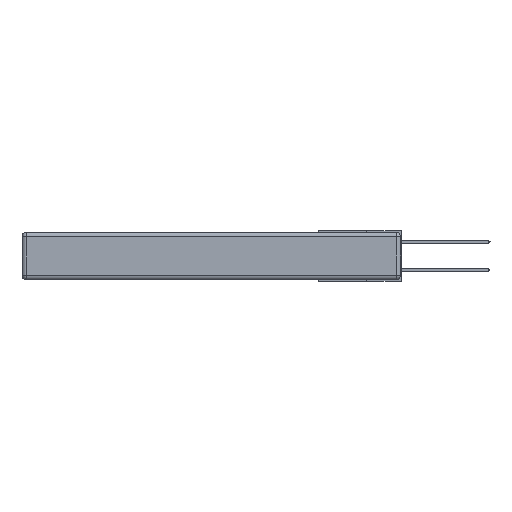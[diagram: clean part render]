
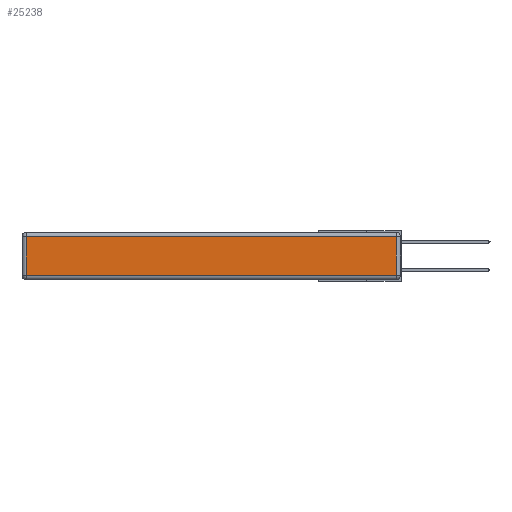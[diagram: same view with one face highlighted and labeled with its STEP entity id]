
A CAD part, left-side view. The second image highlights one B-rep face of the part: STEP entity #25238.
In plain terms, the highlighted planar face has unit normal (-1, 0, 0).
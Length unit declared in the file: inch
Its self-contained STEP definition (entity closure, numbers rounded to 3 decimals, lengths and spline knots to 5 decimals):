
#704 = AXIS2_PLACEMENT_3D ( 'NONE', #15070, #11145, #9154 ) ;
#1471 = VERTEX_POINT ( 'NONE', #9266 ) ;
#2632 = EDGE_LOOP ( 'NONE', ( #19724, #6106, #23826, #5443 ) ) ;
#4002 = VECTOR ( 'NONE', #16890, 39.37008 ) ;
#4607 = LINE ( 'NONE', #25486, #22630 ) ;
#4851 = CARTESIAN_POINT ( 'NONE',  ( 0., 2.72, -0.343 ) ) ;
#5285 = CARTESIAN_POINT ( 'NONE',  ( 0., 2.72, -0.03 ) ) ;
#5443 = ORIENTED_EDGE ( 'NONE', *, *, #9253, .T. ) ;
#6106 = ORIENTED_EDGE ( 'NONE', *, *, #17578, .T. ) ;
#6885 = DIRECTION ( 'NONE',  ( 0., 0., 1. ) ) ;
#8106 = DIRECTION ( 'NONE',  ( 0., 1., 0. ) ) ;
#9154 = DIRECTION ( 'NONE',  ( 0., 0., 1. ) ) ;
#9253 = EDGE_CURVE ( 'NONE', #11743, #22952, #15229, .T. ) ;
#9266 = CARTESIAN_POINT ( 'NONE',  ( 0., 0.03, -0.313 ) ) ;
#11145 = DIRECTION ( 'NONE',  ( -1., 0., 0. ) ) ;
#11191 = EDGE_CURVE ( 'NONE', #17053, #11743, #20093, .T. ) ;
#11743 = VERTEX_POINT ( 'NONE', #5285 ) ;
#13769 = CARTESIAN_POINT ( 'NONE',  ( 0., 0.03, -0.03 ) ) ;
#13907 = VECTOR ( 'NONE', #6885, 39.37008 ) ;
#14688 = CARTESIAN_POINT ( 'NONE',  ( 0., 2.75, -0.03 ) ) ;
#14799 = VECTOR ( 'NONE', #8106, 39.37008 ) ;
#15070 = CARTESIAN_POINT ( 'NONE',  ( 0., 0., -0.343 ) ) ;
#15229 = LINE ( 'NONE', #4851, #4002 ) ;
#15597 = DIRECTION ( 'NONE',  ( 0., -1., 0. ) ) ;
#16209 = EDGE_CURVE ( 'NONE', #22952, #1471, #4607, .T. ) ;
#16890 = DIRECTION ( 'NONE',  ( 0., 0., -1. ) ) ;
#17053 = VERTEX_POINT ( 'NONE', #13769 ) ;
#17578 = EDGE_CURVE ( 'NONE', #1471, #17053, #21042, .T. ) ;
#19445 = FACE_OUTER_BOUND ( 'NONE', #2632, .T. ) ;
#19724 = ORIENTED_EDGE ( 'NONE', *, *, #16209, .T. ) ;
#20093 = LINE ( 'NONE', #14688, #14799 ) ;
#20175 = CARTESIAN_POINT ( 'NONE',  ( 0., 2.72, -0.313 ) ) ;
#21042 = LINE ( 'NONE', #24396, #13907 ) ;
#21046 = PLANE ( 'NONE',  #704 ) ;
#22630 = VECTOR ( 'NONE', #15597, 39.37008 ) ;
#22952 = VERTEX_POINT ( 'NONE', #20175 ) ;
#23826 = ORIENTED_EDGE ( 'NONE', *, *, #11191, .T. ) ;
#24396 = CARTESIAN_POINT ( 'NONE',  ( 0., 0.03, -0.343 ) ) ;
#25238 = ADVANCED_FACE ( 'NONE', ( #19445 ), #21046, .T. ) ;
#25486 = CARTESIAN_POINT ( 'NONE',  ( 0., 0., -0.313 ) ) ;
